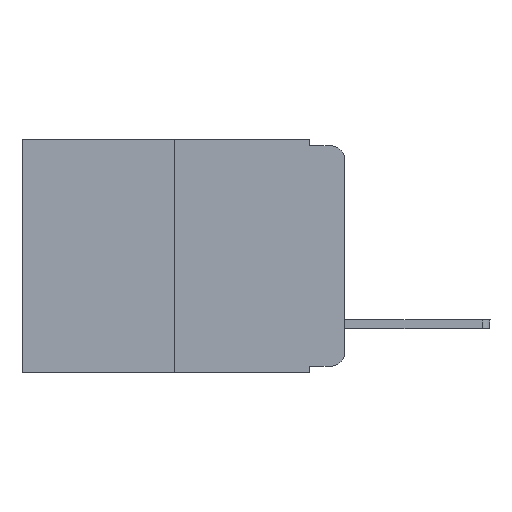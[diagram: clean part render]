
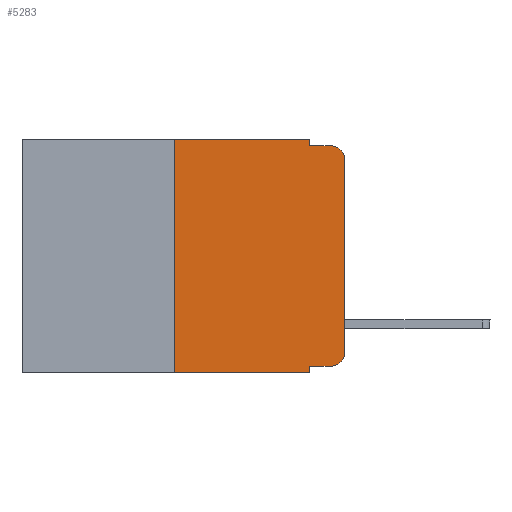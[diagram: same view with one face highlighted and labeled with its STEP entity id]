
A CAD part, left-side view. The second image highlights one B-rep face of the part: STEP entity #5283.
In plain terms, the highlighted planar face has unit normal (-1, 0, 0).
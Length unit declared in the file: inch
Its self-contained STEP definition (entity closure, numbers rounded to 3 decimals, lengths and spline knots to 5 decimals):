
#86 = EDGE_CURVE ( 'NONE', #4027, #5952, #11441, .T. ) ;
#253 = LINE ( 'NONE', #7406, #1945 ) ;
#257 = DIRECTION ( 'NONE',  ( 0., 0., -1. ) ) ;
#452 = CARTESIAN_POINT ( 'NONE',  ( 0., 0.02, -0.03 ) ) ;
#494 = EDGE_CURVE ( 'NONE', #2204, #8873, #11901, .T. ) ;
#579 = EDGE_LOOP ( 'NONE', ( #1765, #8681, #1081, #12532, #8694, #6461, #10419, #6640, #3468, #8881 ) ) ;
#719 = EDGE_CURVE ( 'NONE', #12160, #2091, #9556, .T. ) ;
#984 = LINE ( 'NONE', #3224, #1755 ) ;
#1081 = ORIENTED_EDGE ( 'NONE', *, *, #8040, .F. ) ;
#1137 = AXIS2_PLACEMENT_3D ( 'NONE', #452, #2371, #10307 ) ;
#1319 = CARTESIAN_POINT ( 'NONE',  ( 0., 0.051, -0.01 ) ) ;
#1331 = CARTESIAN_POINT ( 'NONE',  ( 0., 0.051, 0. ) ) ;
#1727 = DIRECTION ( 'NONE',  ( 0., 0., 1. ) ) ;
#1755 = VECTOR ( 'NONE', #10112, 39.37008 ) ;
#1765 = ORIENTED_EDGE ( 'NONE', *, *, #9292, .T. ) ;
#1945 = VECTOR ( 'NONE', #6542, 39.37008 ) ;
#2091 = VERTEX_POINT ( 'NONE', #6878 ) ;
#2139 = CARTESIAN_POINT ( 'NONE',  ( 0., 0.051, -0.333 ) ) ;
#2154 = CARTESIAN_POINT ( 'NONE',  ( 0., 0.25, -0.343 ) ) ;
#2204 = VERTEX_POINT ( 'NONE', #2139 ) ;
#2345 = CARTESIAN_POINT ( 'NONE',  ( 0., 0.051, 0. ) ) ;
#2371 = DIRECTION ( 'NONE',  ( -1., 0., 0. ) ) ;
#2832 = CARTESIAN_POINT ( 'NONE',  ( 0., 0.25, 0. ) ) ;
#3224 = CARTESIAN_POINT ( 'NONE',  ( 0., 0., 0. ) ) ;
#3468 = ORIENTED_EDGE ( 'NONE', *, *, #494, .T. ) ;
#3505 = LINE ( 'NONE', #7102, #11131 ) ;
#4027 = VERTEX_POINT ( 'NONE', #12908 ) ;
#4910 = DIRECTION ( 'NONE',  ( 0., -1., 0. ) ) ;
#5156 = DIRECTION ( 'NONE',  ( 0., -1., 0. ) ) ;
#5240 = DIRECTION ( 'NONE',  ( 1., 0., 0. ) ) ;
#5283 = ADVANCED_FACE ( 'NONE', ( #5506 ), #11196, .F. ) ;
#5441 = CARTESIAN_POINT ( 'NONE',  ( 0., 0.051, -0.343 ) ) ;
#5506 = FACE_OUTER_BOUND ( 'NONE', #579, .T. ) ;
#5798 = EDGE_CURVE ( 'NONE', #8657, #4027, #3505, .T. ) ;
#5952 = VERTEX_POINT ( 'NONE', #1319 ) ;
#6268 = CARTESIAN_POINT ( 'NONE',  ( 0., 0.02, -0.333 ) ) ;
#6354 = AXIS2_PLACEMENT_3D ( 'NONE', #8726, #6678, #10741 ) ;
#6365 = CARTESIAN_POINT ( 'NONE',  ( 0., 0., -0.313 ) ) ;
#6368 = VECTOR ( 'NONE', #5156, 39.37008 ) ;
#6461 = ORIENTED_EDGE ( 'NONE', *, *, #10671, .F. ) ;
#6542 = DIRECTION ( 'NONE',  ( 0., -1., 0. ) ) ;
#6640 = ORIENTED_EDGE ( 'NONE', *, *, #7920, .F. ) ;
#6678 = DIRECTION ( 'NONE',  ( -1., 0., 0. ) ) ;
#6878 = CARTESIAN_POINT ( 'NONE',  ( 0., 0.02, -0.01 ) ) ;
#6890 = EDGE_CURVE ( 'NONE', #9773, #12388, #10874, .T. ) ;
#6940 = CARTESIAN_POINT ( 'NONE',  ( 0., 0.051, -0.333 ) ) ;
#7102 = CARTESIAN_POINT ( 'NONE',  ( 0., 0.473, 0. ) ) ;
#7186 = EDGE_CURVE ( 'NONE', #8873, #11124, #8378, .T. ) ;
#7406 = CARTESIAN_POINT ( 'NONE',  ( 0., 0.051, -0.01 ) ) ;
#7818 = VECTOR ( 'NONE', #1727, 39.37008 ) ;
#7920 = EDGE_CURVE ( 'NONE', #2204, #12388, #10078, .T. ) ;
#8013 = VECTOR ( 'NONE', #8237, 39.37008 ) ;
#8040 = EDGE_CURVE ( 'NONE', #5952, #2091, #253, .T. ) ;
#8237 = DIRECTION ( 'NONE',  ( 0., 0., -1. ) ) ;
#8378 = CIRCLE ( 'NONE', #6354, 0.02 ) ;
#8657 = VERTEX_POINT ( 'NONE', #10437 ) ;
#8681 = ORIENTED_EDGE ( 'NONE', *, *, #719, .T. ) ;
#8694 = ORIENTED_EDGE ( 'NONE', *, *, #5798, .F. ) ;
#8726 = CARTESIAN_POINT ( 'NONE',  ( 0., 0.02, -0.313 ) ) ;
#8873 = VERTEX_POINT ( 'NONE', #6268 ) ;
#8881 = ORIENTED_EDGE ( 'NONE', *, *, #7186, .T. ) ;
#8903 = CARTESIAN_POINT ( 'NONE',  ( 0., 0.473, -0.343 ) ) ;
#9181 = DIRECTION ( 'NONE',  ( 0., -1., 0. ) ) ;
#9292 = EDGE_CURVE ( 'NONE', #11124, #12160, #984, .T. ) ;
#9556 = CIRCLE ( 'NONE', #1137, 0.02 ) ;
#9773 = VERTEX_POINT ( 'NONE', #2154 ) ;
#10020 = VECTOR ( 'NONE', #4910, 39.37008 ) ;
#10078 = LINE ( 'NONE', #1331, #12892 ) ;
#10112 = DIRECTION ( 'NONE',  ( 0., 0., 1. ) ) ;
#10278 = CARTESIAN_POINT ( 'NONE',  ( 0., 0.473, 0. ) ) ;
#10307 = DIRECTION ( 'NONE',  ( 0., 0., -1. ) ) ;
#10419 = ORIENTED_EDGE ( 'NONE', *, *, #6890, .T. ) ;
#10437 = CARTESIAN_POINT ( 'NONE',  ( 0., 0.25, 0. ) ) ;
#10465 = LINE ( 'NONE', #2832, #7818 ) ;
#10671 = EDGE_CURVE ( 'NONE', #9773, #8657, #10465, .T. ) ;
#10741 = DIRECTION ( 'NONE',  ( 0., 0., -1. ) ) ;
#10874 = LINE ( 'NONE', #8903, #6368 ) ;
#11124 = VERTEX_POINT ( 'NONE', #6365 ) ;
#11131 = VECTOR ( 'NONE', #9181, 39.37008 ) ;
#11196 = PLANE ( 'NONE',  #12105 ) ;
#11230 = DIRECTION ( 'NONE',  ( 0., 0., -1. ) ) ;
#11441 = LINE ( 'NONE', #2345, #8013 ) ;
#11901 = LINE ( 'NONE', #6940, #10020 ) ;
#11970 = CARTESIAN_POINT ( 'NONE',  ( 0., 0., -0.03 ) ) ;
#12105 = AXIS2_PLACEMENT_3D ( 'NONE', #10278, #5240, #257 ) ;
#12160 = VERTEX_POINT ( 'NONE', #11970 ) ;
#12388 = VERTEX_POINT ( 'NONE', #5441 ) ;
#12532 = ORIENTED_EDGE ( 'NONE', *, *, #86, .F. ) ;
#12892 = VECTOR ( 'NONE', #11230, 39.37008 ) ;
#12908 = CARTESIAN_POINT ( 'NONE',  ( 0., 0.051, 0. ) ) ;
